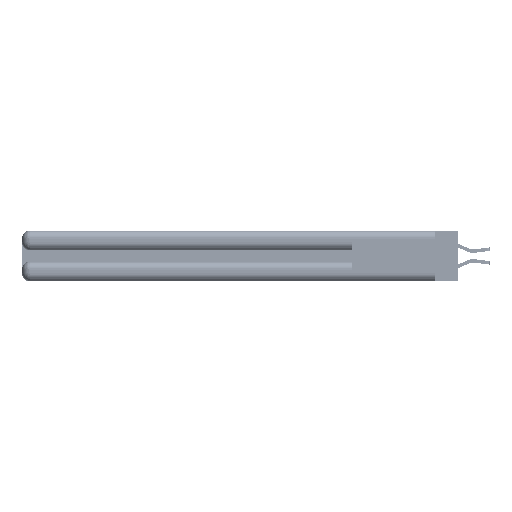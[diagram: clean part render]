
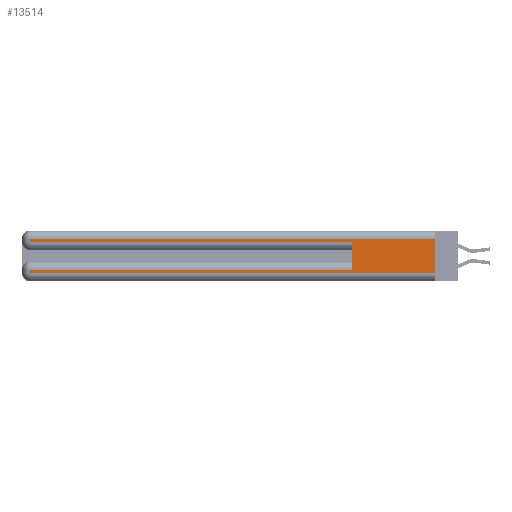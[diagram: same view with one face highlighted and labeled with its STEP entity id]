
A CAD part, left-side view. The second image highlights one B-rep face of the part: STEP entity #13514.
In plain terms, the highlighted planar face has unit normal (-1, 0, 0).
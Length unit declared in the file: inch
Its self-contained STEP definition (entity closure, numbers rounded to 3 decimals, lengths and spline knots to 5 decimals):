
#29 = DIRECTION ( 'NONE',  ( 0., 0., -1. ) ) ;
#726 = CARTESIAN_POINT ( 'NONE',  ( 0., 0., 0.06 ) ) ;
#1102 = EDGE_CURVE ( 'NONE', #38640, #33525, #23496, .T. ) ;
#1526 = DIRECTION ( 'NONE',  ( 0., -1., 0. ) ) ;
#1627 = ORIENTED_EDGE ( 'NONE', *, *, #1102, .F. ) ;
#1823 = LINE ( 'NONE', #18435, #32650 ) ;
#1945 = ORIENTED_EDGE ( 'NONE', *, *, #15048, .F. ) ;
#1963 = DIRECTION ( 'NONE',  ( 0., 1., 0. ) ) ;
#2811 = VERTEX_POINT ( 'NONE', #21577 ) ;
#3277 = VECTOR ( 'NONE', #10091, 39.37008 ) ;
#3669 = EDGE_LOOP ( 'NONE', ( #1945, #11924, #27735, #20501, #1627, #25942, #26474, #9577 ) ) ;
#5736 = CARTESIAN_POINT ( 'NONE',  ( 0., 2.94, 0.085 ) ) ;
#6388 = VECTOR ( 'NONE', #1963, 39.37008 ) ;
#6541 = PLANE ( 'NONE',  #10653 ) ;
#6635 = LINE ( 'NONE', #10238, #14300 ) ;
#6836 = CARTESIAN_POINT ( 'NONE',  ( 0., 0., 0.085 ) ) ;
#7110 = EDGE_CURVE ( 'NONE', #18009, #33525, #32839, .T. ) ;
#7371 = DIRECTION ( 'NONE',  ( 0., -1., 0. ) ) ;
#7607 = EDGE_CURVE ( 'NONE', #21465, #33127, #6635, .T. ) ;
#7626 = VECTOR ( 'NONE', #7371, 39.37008 ) ;
#7914 = CARTESIAN_POINT ( 'NONE',  ( 0., 0.6, 0.285 ) ) ;
#8682 = EDGE_CURVE ( 'NONE', #42391, #18009, #20754, .T. ) ;
#9577 = ORIENTED_EDGE ( 'NONE', *, *, #38224, .T. ) ;
#10091 = DIRECTION ( 'NONE',  ( 0., 1., 0. ) ) ;
#10238 = CARTESIAN_POINT ( 'NONE',  ( 0., 2.94, 0.37 ) ) ;
#10653 = AXIS2_PLACEMENT_3D ( 'NONE', #39372, #19705, #29 ) ;
#11924 = ORIENTED_EDGE ( 'NONE', *, *, #20841, .T. ) ;
#12472 = CARTESIAN_POINT ( 'NONE',  ( 0., 0.6, 0.085 ) ) ;
#13514 = ADVANCED_FACE ( 'NONE', ( #29161 ), #6541, .F. ) ;
#14300 = VECTOR ( 'NONE', #23444, 39.37008 ) ;
#15048 = EDGE_CURVE ( 'NONE', #34136, #2811, #1823, .T. ) ;
#15156 = DIRECTION ( 'NONE',  ( 0., 0., -1. ) ) ;
#15391 = VECTOR ( 'NONE', #1526, 39.37008 ) ;
#18009 = VERTEX_POINT ( 'NONE', #34114 ) ;
#18311 = DIRECTION ( 'NONE',  ( 0., 0., 1. ) ) ;
#18435 = CARTESIAN_POINT ( 'NONE',  ( 0., 0., 0.37 ) ) ;
#19705 = DIRECTION ( 'NONE',  ( 1., 0., 0. ) ) ;
#20501 = ORIENTED_EDGE ( 'NONE', *, *, #7110, .T. ) ;
#20754 = LINE ( 'NONE', #22782, #38257 ) ;
#20841 = EDGE_CURVE ( 'NONE', #34136, #42391, #41258, .T. ) ;
#21465 = VERTEX_POINT ( 'NONE', #5736 ) ;
#21577 = CARTESIAN_POINT ( 'NONE',  ( 0., 0., 0.06 ) ) ;
#22348 = EDGE_CURVE ( 'NONE', #38640, #21465, #29458, .T. ) ;
#22782 = CARTESIAN_POINT ( 'NONE',  ( 0., 2.94, 0.37 ) ) ;
#23444 = DIRECTION ( 'NONE',  ( 0., 0., -1. ) ) ;
#23496 = LINE ( 'NONE', #28068, #39930 ) ;
#24039 = CARTESIAN_POINT ( 'NONE',  ( 0., 0., 0.31 ) ) ;
#25050 = LINE ( 'NONE', #726, #7626 ) ;
#25942 = ORIENTED_EDGE ( 'NONE', *, *, #22348, .T. ) ;
#26474 = ORIENTED_EDGE ( 'NONE', *, *, #7607, .T. ) ;
#26539 = CARTESIAN_POINT ( 'NONE',  ( 0., 2.94, 0.31 ) ) ;
#27735 = ORIENTED_EDGE ( 'NONE', *, *, #8682, .T. ) ;
#28068 = CARTESIAN_POINT ( 'NONE',  ( 0., 0.6, 0.145 ) ) ;
#28204 = CARTESIAN_POINT ( 'NONE',  ( 0., 0., 0.31 ) ) ;
#28414 = CARTESIAN_POINT ( 'NONE',  ( 0., 2.94, 0.06 ) ) ;
#29161 = FACE_OUTER_BOUND ( 'NONE', #3669, .T. ) ;
#29458 = LINE ( 'NONE', #6836, #3277 ) ;
#32587 = DIRECTION ( 'NONE',  ( 0., 0., -1. ) ) ;
#32650 = VECTOR ( 'NONE', #15156, 39.37008 ) ;
#32839 = LINE ( 'NONE', #40846, #15391 ) ;
#33127 = VERTEX_POINT ( 'NONE', #28414 ) ;
#33525 = VERTEX_POINT ( 'NONE', #7914 ) ;
#34114 = CARTESIAN_POINT ( 'NONE',  ( 0., 2.94, 0.285 ) ) ;
#34136 = VERTEX_POINT ( 'NONE', #24039 ) ;
#38224 = EDGE_CURVE ( 'NONE', #33127, #2811, #25050, .T. ) ;
#38257 = VECTOR ( 'NONE', #32587, 39.37008 ) ;
#38640 = VERTEX_POINT ( 'NONE', #12472 ) ;
#39372 = CARTESIAN_POINT ( 'NONE',  ( 0., 0., 0.37 ) ) ;
#39930 = VECTOR ( 'NONE', #18311, 39.37008 ) ;
#40846 = CARTESIAN_POINT ( 'NONE',  ( 0., 0., 0.285 ) ) ;
#41258 = LINE ( 'NONE', #28204, #6388 ) ;
#42391 = VERTEX_POINT ( 'NONE', #26539 ) ;
